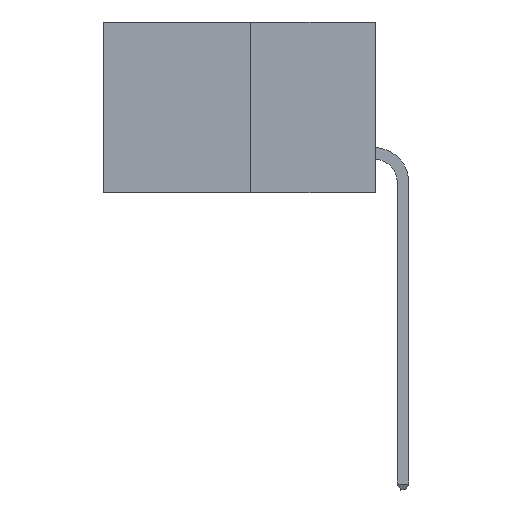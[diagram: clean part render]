
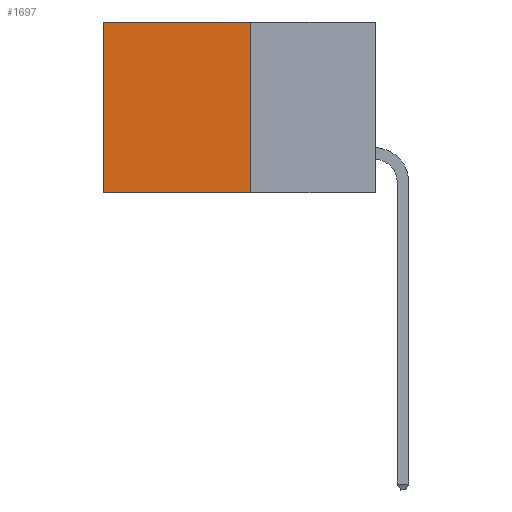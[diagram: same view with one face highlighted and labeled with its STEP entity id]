
A CAD part, left-side view. The second image highlights one B-rep face of the part: STEP entity #1697.
In plain terms, the highlighted planar face has unit normal (-1, 0, 0).
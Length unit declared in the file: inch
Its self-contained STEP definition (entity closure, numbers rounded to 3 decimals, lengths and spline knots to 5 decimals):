
#656 = EDGE_CURVE ( 'NONE', #12645, #9068, #7517, .T. ) ;
#746 = CARTESIAN_POINT ( 'NONE',  ( 0.277, 0.27, -0.37 ) ) ;
#789 = EDGE_LOOP ( 'NONE', ( #15384, #12243, #4640, #2065 ) ) ;
#1697 = ADVANCED_FACE ( 'NONE', ( #15641 ), #14462, .F. ) ;
#1909 = CARTESIAN_POINT ( 'NONE',  ( 0.277, 0.27, 0. ) ) ;
#2065 = ORIENTED_EDGE ( 'NONE', *, *, #5942, .T. ) ;
#2843 = VERTEX_POINT ( 'NONE', #1909 ) ;
#4161 = CARTESIAN_POINT ( 'NONE',  ( 0.277, 0.27, 0. ) ) ;
#4307 = LINE ( 'NONE', #4161, #13970 ) ;
#4313 = CARTESIAN_POINT ( 'NONE',  ( 0.277, 0.59, -0.37 ) ) ;
#4640 = ORIENTED_EDGE ( 'NONE', *, *, #5735, .F. ) ;
#4821 = AXIS2_PLACEMENT_3D ( 'NONE', #13639, #13586, #13831 ) ;
#5735 = EDGE_CURVE ( 'NONE', #2843, #10227, #7866, .T. ) ;
#5942 = EDGE_CURVE ( 'NONE', #2843, #12645, #4307, .T. ) ;
#7067 = VECTOR ( 'NONE', #15891, 39.37008 ) ;
#7517 = LINE ( 'NONE', #11863, #10332 ) ;
#7648 = EDGE_CURVE ( 'NONE', #10227, #9068, #12608, .T. ) ;
#7866 = LINE ( 'NONE', #14686, #7067 ) ;
#7900 = DIRECTION ( 'NONE',  ( 0., 1., 0. ) ) ;
#9068 = VERTEX_POINT ( 'NONE', #4313 ) ;
#10227 = VERTEX_POINT ( 'NONE', #11505 ) ;
#10332 = VECTOR ( 'NONE', #11616, 39.37008 ) ;
#11505 = CARTESIAN_POINT ( 'NONE',  ( 0.277, 0.27, -0.37 ) ) ;
#11616 = DIRECTION ( 'NONE',  ( 0., 0., -1. ) ) ;
#11863 = CARTESIAN_POINT ( 'NONE',  ( 0.277, 0.59, -0.37 ) ) ;
#12243 = ORIENTED_EDGE ( 'NONE', *, *, #7648, .F. ) ;
#12608 = LINE ( 'NONE', #746, #15018 ) ;
#12645 = VERTEX_POINT ( 'NONE', #15708 ) ;
#13078 = DIRECTION ( 'NONE',  ( 0., 1., 0. ) ) ;
#13586 = DIRECTION ( 'NONE',  ( 1., 0., 0. ) ) ;
#13639 = CARTESIAN_POINT ( 'NONE',  ( 0.277, 0.27, -0.37 ) ) ;
#13831 = DIRECTION ( 'NONE',  ( 0., 0., -1. ) ) ;
#13970 = VECTOR ( 'NONE', #7900, 39.37008 ) ;
#14462 = PLANE ( 'NONE',  #4821 ) ;
#14686 = CARTESIAN_POINT ( 'NONE',  ( 0.277, 0.27, -0.37 ) ) ;
#15018 = VECTOR ( 'NONE', #13078, 39.37008 ) ;
#15384 = ORIENTED_EDGE ( 'NONE', *, *, #656, .T. ) ;
#15641 = FACE_OUTER_BOUND ( 'NONE', #789, .T. ) ;
#15708 = CARTESIAN_POINT ( 'NONE',  ( 0.277, 0.59, 0. ) ) ;
#15891 = DIRECTION ( 'NONE',  ( 0., 0., -1. ) ) ;
